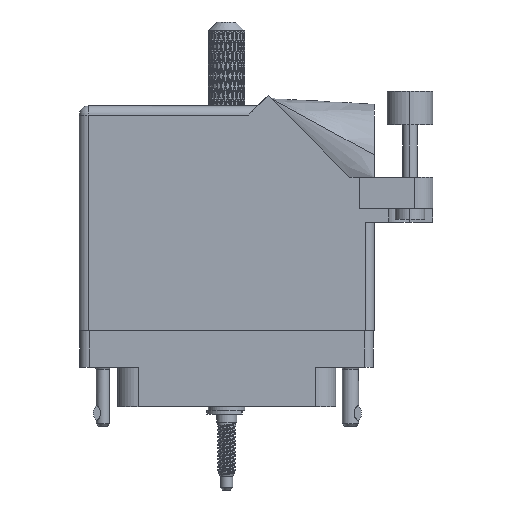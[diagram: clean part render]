
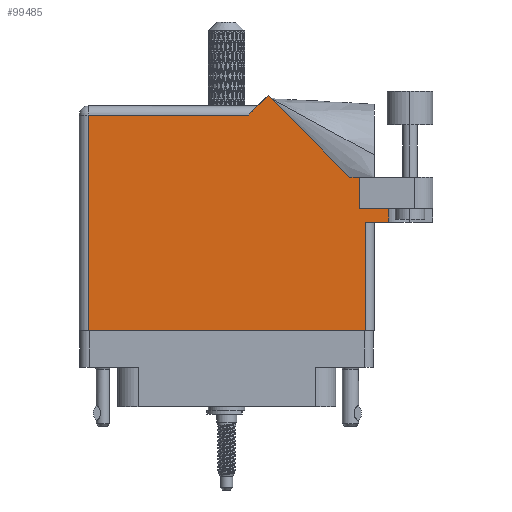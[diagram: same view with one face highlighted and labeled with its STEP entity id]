
A CAD part, front view. The second image highlights one B-rep face of the part: STEP entity #99485.
In plain terms, the highlighted face is planar.
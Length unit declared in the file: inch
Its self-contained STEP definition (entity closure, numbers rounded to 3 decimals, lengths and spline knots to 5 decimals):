
#633 = VECTOR ( 'NONE', #89682, 39.37008 ) ;
#2530 = CARTESIAN_POINT ( 'NONE',  ( -0.943, 1.368, 0.455 ) ) ;
#2585 = DIRECTION ( 'NONE',  ( -1., 0., 0. ) ) ;
#2674 = LINE ( 'NONE', #58826, #102976 ) ;
#3498 = DIRECTION ( 'NONE',  ( 0., 1., 0. ) ) ;
#5531 = VECTOR ( 'NONE', #107282, 39.37008 ) ;
#10405 = VECTOR ( 'NONE', #3498, 39.37008 ) ;
#11659 = LINE ( 'NONE', #83069, #103577 ) ;
#11784 = CARTESIAN_POINT ( 'NONE',  ( 1.1065, 0.731, 0.455 ) ) ;
#17438 = LINE ( 'NONE', #55389, #633 ) ;
#17444 = ORIENTED_EDGE ( 'NONE', *, *, #94718, .T. ) ;
#19837 = CARTESIAN_POINT ( 'NONE',  ( 0.28271, 1.50071, 0.455 ) ) ;
#20075 = DIRECTION ( 'NONE',  ( 0., 0., -1. ) ) ;
#22437 = DIRECTION ( 'NONE',  ( 1., 0., 0. ) ) ;
#22884 = ORIENTED_EDGE ( 'NONE', *, *, #83945, .F. ) ;
#22976 = VERTEX_POINT ( 'NONE', #31479 ) ;
#23529 = CARTESIAN_POINT ( 'NONE',  ( 0.212, 1.43, 0.455 ) ) ;
#27496 = CARTESIAN_POINT ( 'NONE',  ( 0.83942, 0.944, 0.455 ) ) ;
#29709 = DIRECTION ( 'NONE',  ( 0., 1., 0. ) ) ;
#31479 = CARTESIAN_POINT ( 'NONE',  ( 0.905, 0.944, 0.455 ) ) ;
#32876 = EDGE_CURVE ( 'NONE', #68669, #88978, #101587, .T. ) ;
#33970 = ORIENTED_EDGE ( 'NONE', *, *, #53785, .T. ) ;
#36491 = ORIENTED_EDGE ( 'NONE', *, *, #89107, .T. ) ;
#36848 = DIRECTION ( 'NONE',  ( -1., 0., 0. ) ) ;
#37702 = ORIENTED_EDGE ( 'NONE', *, *, #38287, .T. ) ;
#38287 = EDGE_CURVE ( 'NONE', #84572, #99973, #17438, .T. ) ;
#39168 = ORIENTED_EDGE ( 'NONE', *, *, #32876, .T. ) ;
#42872 = ORIENTED_EDGE ( 'NONE', *, *, #45662, .T. ) ;
#45039 = EDGE_LOOP ( 'NONE', ( #17444, #60278, #56352, #82007, #22884, #36491, #42872, #39168, #33970, #80798, #37702 ) ) ;
#45662 = EDGE_CURVE ( 'NONE', #22976, #68669, #64698, .T. ) ;
#45671 = FACE_OUTER_BOUND ( 'NONE', #45039, .T. ) ;
#48151 = LINE ( 'NONE', #50166, #102644 ) ;
#48387 = CARTESIAN_POINT ( 'NONE',  ( -1.005, 1.43, 0.455 ) ) ;
#48506 = DIRECTION ( 'NONE',  ( 1., 0., 0. ) ) ;
#49535 = VERTEX_POINT ( 'NONE', #61681 ) ;
#50025 = CARTESIAN_POINT ( 'NONE',  ( 1.005, 0.637, 0.455 ) ) ;
#50166 = CARTESIAN_POINT ( 'NONE',  ( 0.905, 0.731, 0.455 ) ) ;
#50208 = CARTESIAN_POINT ( 'NONE',  ( 0.905, 0.731, 0.455 ) ) ;
#50297 = EDGE_CURVE ( 'NONE', #56760, #84572, #2674, .T. ) ;
#51742 = CARTESIAN_POINT ( 'NONE',  ( 0.15, 1.368, 0.455 ) ) ;
#53785 = EDGE_CURVE ( 'NONE', #88978, #56760, #82833, .T. ) ;
#55389 = CARTESIAN_POINT ( 'NONE',  ( -0.943, -0.1, 0.455 ) ) ;
#55939 = EDGE_CURVE ( 'NONE', #94209, #79090, #96381, .T. ) ;
#56352 = ORIENTED_EDGE ( 'NONE', *, *, #96310, .T. ) ;
#56760 = VERTEX_POINT ( 'NONE', #51742 ) ;
#57529 = CARTESIAN_POINT ( 'NONE',  ( 0.905, 0.731, 0.455 ) ) ;
#58248 = CARTESIAN_POINT ( 'NONE',  ( 1.1065, 1.06177, 0.455 ) ) ;
#58646 = LINE ( 'NONE', #50025, #89308 ) ;
#58826 = CARTESIAN_POINT ( 'NONE',  ( -1.005, 1.368, 0.455 ) ) ;
#59638 = VECTOR ( 'NONE', #48506, 39.37008 ) ;
#60278 = ORIENTED_EDGE ( 'NONE', *, *, #90465, .T. ) ;
#61681 = CARTESIAN_POINT ( 'NONE',  ( 0.943, 0.637, 0.455 ) ) ;
#64698 = LINE ( 'NONE', #90653, #106542 ) ;
#65205 = CARTESIAN_POINT ( 'NONE',  ( 1.1065, 0.637, 0.455 ) ) ;
#68669 = VERTEX_POINT ( 'NONE', #106698 ) ;
#74988 = LINE ( 'NONE', #110460, #59638 ) ;
#78974 = VERTEX_POINT ( 'NONE', #107334 ) ;
#79090 = VERTEX_POINT ( 'NONE', #65205 ) ;
#79655 = VERTEX_POINT ( 'NONE', #50208 ) ;
#80798 = ORIENTED_EDGE ( 'NONE', *, *, #50297, .T. ) ;
#82007 = ORIENTED_EDGE ( 'NONE', *, *, #55939, .F. ) ;
#82377 = PLANE ( 'NONE',  #101298 ) ;
#82833 = LINE ( 'NONE', #23529, #96811 ) ;
#83069 = CARTESIAN_POINT ( 'NONE',  ( 0.943, 0.637, 0.455 ) ) ;
#83945 = EDGE_CURVE ( 'NONE', #79655, #94209, #48151, .T. ) ;
#84572 = VERTEX_POINT ( 'NONE', #2530 ) ;
#86898 = DIRECTION ( 'NONE',  ( -1., 0., 0. ) ) ;
#88978 = VERTEX_POINT ( 'NONE', #19837 ) ;
#89107 = EDGE_CURVE ( 'NONE', #79655, #22976, #99581, .T. ) ;
#89308 = VECTOR ( 'NONE', #22437, 39.37008 ) ;
#89682 = DIRECTION ( 'NONE',  ( 0., -1., 0. ) ) ;
#90465 = EDGE_CURVE ( 'NONE', #78974, #49535, #11659, .T. ) ;
#90653 = CARTESIAN_POINT ( 'NONE',  ( 1.405, 0.944, 0.455 ) ) ;
#92191 = VECTOR ( 'NONE', #102671, 39.37008 ) ;
#94209 = VERTEX_POINT ( 'NONE', #11784 ) ;
#94718 = EDGE_CURVE ( 'NONE', #99973, #78974, #74988, .T. ) ;
#96310 = EDGE_CURVE ( 'NONE', #49535, #79090, #58646, .T. ) ;
#96381 = LINE ( 'NONE', #58248, #92191 ) ;
#96811 = VECTOR ( 'NONE', #111884, 39.37008 ) ;
#99485 = ADVANCED_FACE ( 'NONE', ( #45671 ), #82377, .F. ) ;
#99581 = LINE ( 'NONE', #57529, #10405 ) ;
#99973 = VERTEX_POINT ( 'NONE', #105569 ) ;
#101298 = AXIS2_PLACEMENT_3D ( 'NONE', #48387, #20075, #2585 ) ;
#101587 = LINE ( 'NONE', #27496, #5531 ) ;
#102644 = VECTOR ( 'NONE', #112462, 39.37008 ) ;
#102671 = DIRECTION ( 'NONE',  ( 0., -1., 0. ) ) ;
#102976 = VECTOR ( 'NONE', #86898, 39.37008 ) ;
#103577 = VECTOR ( 'NONE', #29709, 39.37008 ) ;
#105569 = CARTESIAN_POINT ( 'NONE',  ( -0.943, -0.1, 0.455 ) ) ;
#106542 = VECTOR ( 'NONE', #36848, 39.37008 ) ;
#106698 = CARTESIAN_POINT ( 'NONE',  ( 0.83942, 0.944, 0.455 ) ) ;
#107282 = DIRECTION ( 'NONE',  ( -0.707, 0.707, 0. ) ) ;
#107334 = CARTESIAN_POINT ( 'NONE',  ( 0.943, -0.1, 0.455 ) ) ;
#110460 = CARTESIAN_POINT ( 'NONE',  ( -1.005, -0.1, 0.455 ) ) ;
#111884 = DIRECTION ( 'NONE',  ( -0.707, -0.707, 0. ) ) ;
#112462 = DIRECTION ( 'NONE',  ( 1., 0., 0. ) ) ;
